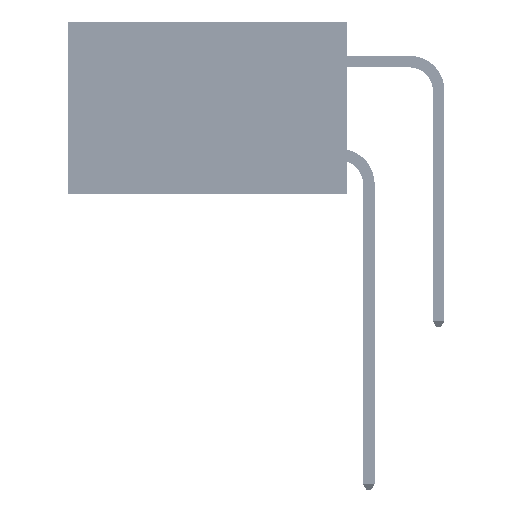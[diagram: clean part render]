
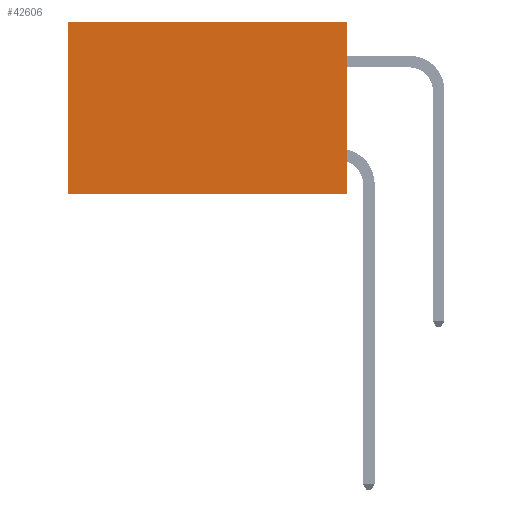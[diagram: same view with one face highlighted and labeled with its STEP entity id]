
A CAD part, left-side view. The second image highlights one B-rep face of the part: STEP entity #42606.
In plain terms, the highlighted planar face has unit normal (-1, 0, 0).
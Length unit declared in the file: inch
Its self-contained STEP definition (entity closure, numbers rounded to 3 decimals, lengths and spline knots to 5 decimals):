
#996 = EDGE_CURVE ( 'NONE', #8879, #42144, #30541, .T. ) ;
#2128 = VECTOR ( 'NONE', #17639, 39.37008 ) ;
#2829 = VECTOR ( 'NONE', #36409, 39.37008 ) ;
#3738 = PLANE ( 'NONE',  #29426 ) ;
#7034 = VERTEX_POINT ( 'NONE', #24504 ) ;
#7561 = DIRECTION ( 'NONE',  ( 1., 0., 0. ) ) ;
#8879 = VERTEX_POINT ( 'NONE', #16751 ) ;
#10817 = VECTOR ( 'NONE', #30694, 39.37008 ) ;
#12710 = CARTESIAN_POINT ( 'NONE',  ( 0.2875, 0., -0.37 ) ) ;
#14280 = CARTESIAN_POINT ( 'NONE',  ( 0.2875, 0., 0. ) ) ;
#15473 = FACE_OUTER_BOUND ( 'NONE', #38144, .T. ) ;
#16751 = CARTESIAN_POINT ( 'NONE',  ( 0.2875, 0., -0.37 ) ) ;
#17639 = DIRECTION ( 'NONE',  ( 0., 0., -1. ) ) ;
#18395 = EDGE_CURVE ( 'NONE', #7034, #42144, #29402, .T. ) ;
#18559 = ORIENTED_EDGE ( 'NONE', *, *, #996, .F. ) ;
#21538 = LINE ( 'NONE', #14280, #2829 ) ;
#21881 = EDGE_CURVE ( 'NONE', #32636, #7034, #21538, .T. ) ;
#23733 = ORIENTED_EDGE ( 'NONE', *, *, #40906, .F. ) ;
#24504 = CARTESIAN_POINT ( 'NONE',  ( 0.2875, 0.6, 0. ) ) ;
#28168 = CARTESIAN_POINT ( 'NONE',  ( 0.2875, 0.6, 0. ) ) ;
#29402 = LINE ( 'NONE', #28168, #47765 ) ;
#29426 = AXIS2_PLACEMENT_3D ( 'NONE', #37023, #7561, #33488 ) ;
#30541 = LINE ( 'NONE', #12710, #10817 ) ;
#30649 = CARTESIAN_POINT ( 'NONE',  ( 0.2875, 0.6, -0.37 ) ) ;
#30694 = DIRECTION ( 'NONE',  ( 0., 1., 0. ) ) ;
#31823 = LINE ( 'NONE', #36030, #2128 ) ;
#32636 = VERTEX_POINT ( 'NONE', #33258 ) ;
#33258 = CARTESIAN_POINT ( 'NONE',  ( 0.2875, 0., 0. ) ) ;
#33488 = DIRECTION ( 'NONE',  ( 0., 0., -1. ) ) ;
#35585 = DIRECTION ( 'NONE',  ( 0., 0., -1. ) ) ;
#36030 = CARTESIAN_POINT ( 'NONE',  ( 0.2875, 0., 0. ) ) ;
#36409 = DIRECTION ( 'NONE',  ( 0., 1., 0. ) ) ;
#37023 = CARTESIAN_POINT ( 'NONE',  ( 0.2875, 0., 0. ) ) ;
#38144 = EDGE_LOOP ( 'NONE', ( #44437, #18559, #23733, #43165 ) ) ;
#40906 = EDGE_CURVE ( 'NONE', #32636, #8879, #31823, .T. ) ;
#42144 = VERTEX_POINT ( 'NONE', #30649 ) ;
#42606 = ADVANCED_FACE ( 'NONE', ( #15473 ), #3738, .F. ) ;
#43165 = ORIENTED_EDGE ( 'NONE', *, *, #21881, .T. ) ;
#44437 = ORIENTED_EDGE ( 'NONE', *, *, #18395, .T. ) ;
#47765 = VECTOR ( 'NONE', #35585, 39.37008 ) ;
